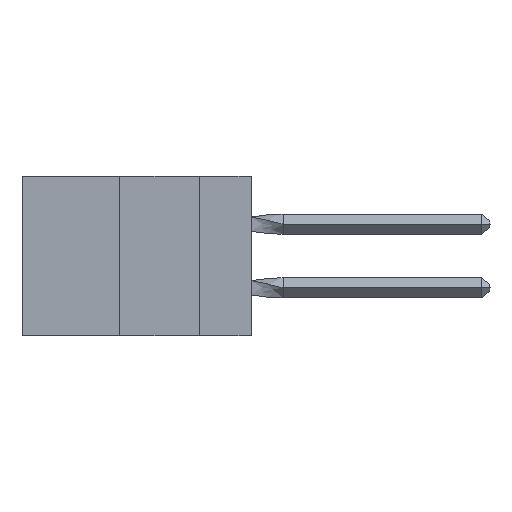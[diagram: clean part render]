
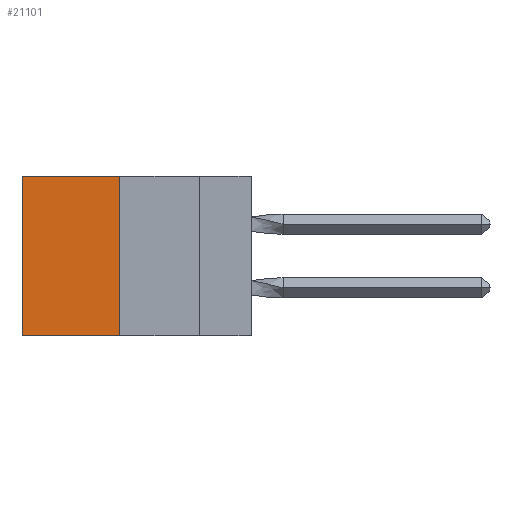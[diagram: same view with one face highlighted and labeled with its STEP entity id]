
A CAD part, left-side view. The second image highlights one B-rep face of the part: STEP entity #21101.
In plain terms, the highlighted planar face has unit normal (-1, 0, 0).
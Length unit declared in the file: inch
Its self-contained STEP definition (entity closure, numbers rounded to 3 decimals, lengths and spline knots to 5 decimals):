
#448 = PLANE ( 'NONE',  #3552 ) ;
#795 = DIRECTION ( 'NONE',  ( 0., 1., 0. ) ) ;
#1110 = EDGE_CURVE ( 'NONE', #16836, #11229, #21954, .T. ) ;
#2090 = DIRECTION ( 'NONE',  ( 1., 0., 0. ) ) ;
#3552 = AXIS2_PLACEMENT_3D ( 'NONE', #17184, #2090, #13348 ) ;
#4228 = CARTESIAN_POINT ( 'NONE',  ( 0.305, 0.413, 0. ) ) ;
#5567 = ORIENTED_EDGE ( 'NONE', *, *, #1110, .T. ) ;
#6083 = DIRECTION ( 'NONE',  ( 0., 1., 0. ) ) ;
#6137 = CARTESIAN_POINT ( 'NONE',  ( 0.305, 0.72, -0.5 ) ) ;
#6985 = VECTOR ( 'NONE', #6083, 39.37008 ) ;
#7782 = VERTEX_POINT ( 'NONE', #9063 ) ;
#9063 = CARTESIAN_POINT ( 'NONE',  ( 0.305, 0.413, 0. ) ) ;
#9564 = DIRECTION ( 'NONE',  ( 0., 0., -1. ) ) ;
#9847 = CARTESIAN_POINT ( 'NONE',  ( 0.305, 0.413, -0.5 ) ) ;
#10598 = VECTOR ( 'NONE', #795, 39.37008 ) ;
#10620 = VECTOR ( 'NONE', #9564, 39.37008 ) ;
#11229 = VERTEX_POINT ( 'NONE', #22473 ) ;
#11501 = EDGE_CURVE ( 'NONE', #7782, #11841, #21873, .T. ) ;
#11841 = VERTEX_POINT ( 'NONE', #9847 ) ;
#11913 = EDGE_CURVE ( 'NONE', #7782, #16836, #22728, .T. ) ;
#12353 = ORIENTED_EDGE ( 'NONE', *, *, #11501, .F. ) ;
#13348 = DIRECTION ( 'NONE',  ( 0., 0., -1. ) ) ;
#13618 = CARTESIAN_POINT ( 'NONE',  ( 0.305, 0.72, 0. ) ) ;
#14464 = ORIENTED_EDGE ( 'NONE', *, *, #16502, .F. ) ;
#14959 = LINE ( 'NONE', #23050, #10598 ) ;
#16365 = VECTOR ( 'NONE', #16371, 39.37008 ) ;
#16371 = DIRECTION ( 'NONE',  ( 0., 0., -1. ) ) ;
#16502 = EDGE_CURVE ( 'NONE', #11841, #11229, #14959, .T. ) ;
#16836 = VERTEX_POINT ( 'NONE', #13618 ) ;
#16890 = FACE_OUTER_BOUND ( 'NONE', #21679, .T. ) ;
#17184 = CARTESIAN_POINT ( 'NONE',  ( 0.305, 0.413, -0.5 ) ) ;
#17395 = ORIENTED_EDGE ( 'NONE', *, *, #11913, .T. ) ;
#19871 = CARTESIAN_POINT ( 'NONE',  ( 0.305, 0.413, -0.5 ) ) ;
#21101 = ADVANCED_FACE ( 'NONE', ( #16890 ), #448, .F. ) ;
#21679 = EDGE_LOOP ( 'NONE', ( #5567, #14464, #12353, #17395 ) ) ;
#21873 = LINE ( 'NONE', #19871, #16365 ) ;
#21954 = LINE ( 'NONE', #6137, #10620 ) ;
#22473 = CARTESIAN_POINT ( 'NONE',  ( 0.305, 0.72, -0.5 ) ) ;
#22728 = LINE ( 'NONE', #4228, #6985 ) ;
#23050 = CARTESIAN_POINT ( 'NONE',  ( 0.305, 0.413, -0.5 ) ) ;
